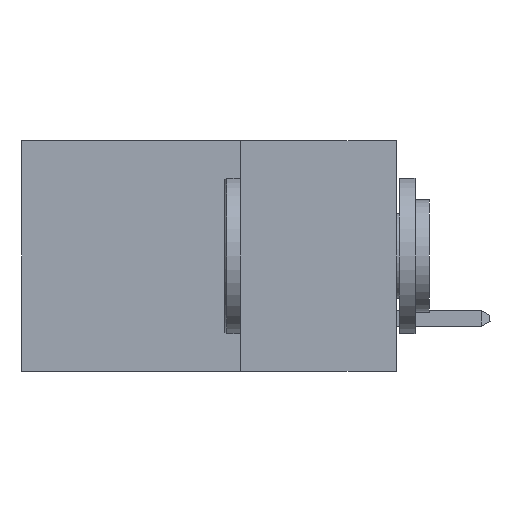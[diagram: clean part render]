
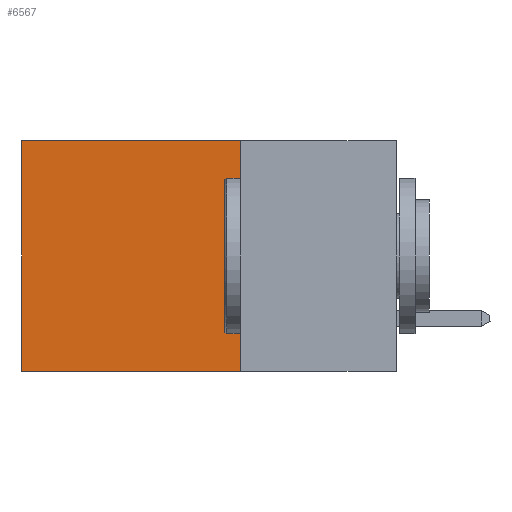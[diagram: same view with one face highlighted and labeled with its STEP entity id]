
A CAD part, left-side view. The second image highlights one B-rep face of the part: STEP entity #6567.
In plain terms, the highlighted planar face has unit normal (-1, 0, 0).
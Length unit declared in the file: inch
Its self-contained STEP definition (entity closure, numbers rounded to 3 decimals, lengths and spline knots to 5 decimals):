
#1774 = EDGE_LOOP ( 'NONE', ( #19030, #16169, #17560, #17461 ) ) ;
#2298 = DIRECTION ( 'NONE',  ( 0., 0., -1. ) ) ;
#3765 = VERTEX_POINT ( 'NONE', #19001 ) ;
#4199 = DIRECTION ( 'NONE',  ( 1., 0., 0. ) ) ;
#4227 = FACE_OUTER_BOUND ( 'NONE', #1774, .T. ) ;
#4372 = VECTOR ( 'NONE', #2298, 39.37008 ) ;
#4476 = CARTESIAN_POINT ( 'NONE',  ( 0.298, 0.25, 0. ) ) ;
#4578 = DIRECTION ( 'NONE',  ( 0., 0., -1. ) ) ;
#5767 = AXIS2_PLACEMENT_3D ( 'NONE', #4476, #4199, #7005 ) ;
#6320 = CARTESIAN_POINT ( 'NONE',  ( 0.298, 0.6, 0. ) ) ;
#6567 = ADVANCED_FACE ( 'NONE', ( #4227 ), #11828, .F. ) ;
#6646 = LINE ( 'NONE', #8802, #11163 ) ;
#7005 = DIRECTION ( 'NONE',  ( 0., 0., -1. ) ) ;
#7931 = EDGE_CURVE ( 'NONE', #21663, #3765, #6646, .T. ) ;
#8199 = LINE ( 'NONE', #18580, #14094 ) ;
#8776 = DIRECTION ( 'NONE',  ( 0., 1., 0. ) ) ;
#8802 = CARTESIAN_POINT ( 'NONE',  ( 0.298, 0.25, -0.37 ) ) ;
#10055 = LINE ( 'NONE', #10948, #4372 ) ;
#10089 = VERTEX_POINT ( 'NONE', #19581 ) ;
#10124 = CARTESIAN_POINT ( 'NONE',  ( 0.298, 0.25, -0.37 ) ) ;
#10948 = CARTESIAN_POINT ( 'NONE',  ( 0.298, 0.6, 0. ) ) ;
#10961 = VERTEX_POINT ( 'NONE', #6320 ) ;
#11163 = VECTOR ( 'NONE', #8776, 39.37008 ) ;
#11828 = PLANE ( 'NONE',  #5767 ) ;
#14094 = VECTOR ( 'NONE', #4578, 39.37008 ) ;
#15728 = LINE ( 'NONE', #18961, #20466 ) ;
#15876 = EDGE_CURVE ( 'NONE', #10089, #21663, #8199, .T. ) ;
#16169 = ORIENTED_EDGE ( 'NONE', *, *, #7931, .F. ) ;
#16853 = EDGE_CURVE ( 'NONE', #10089, #10961, #15728, .T. ) ;
#17461 = ORIENTED_EDGE ( 'NONE', *, *, #16853, .T. ) ;
#17560 = ORIENTED_EDGE ( 'NONE', *, *, #15876, .F. ) ;
#17709 = EDGE_CURVE ( 'NONE', #10961, #3765, #10055, .T. ) ;
#18580 = CARTESIAN_POINT ( 'NONE',  ( 0.298, 0.25, 0. ) ) ;
#18961 = CARTESIAN_POINT ( 'NONE',  ( 0.298, 0.25, 0. ) ) ;
#19001 = CARTESIAN_POINT ( 'NONE',  ( 0.298, 0.6, -0.37 ) ) ;
#19030 = ORIENTED_EDGE ( 'NONE', *, *, #17709, .T. ) ;
#19581 = CARTESIAN_POINT ( 'NONE',  ( 0.298, 0.25, 0. ) ) ;
#20466 = VECTOR ( 'NONE', #20734, 39.37008 ) ;
#20734 = DIRECTION ( 'NONE',  ( 0., 1., 0. ) ) ;
#21663 = VERTEX_POINT ( 'NONE', #10124 ) ;
